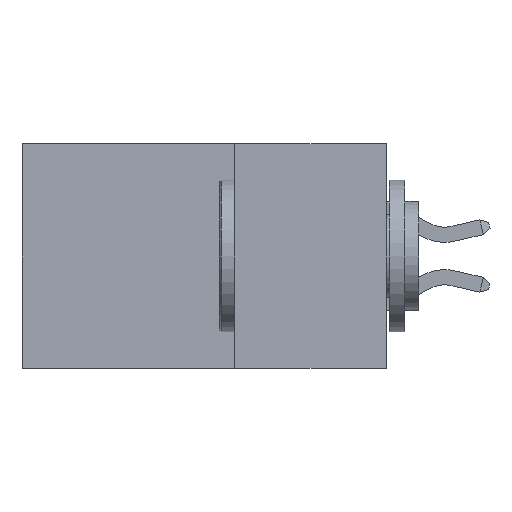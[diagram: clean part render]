
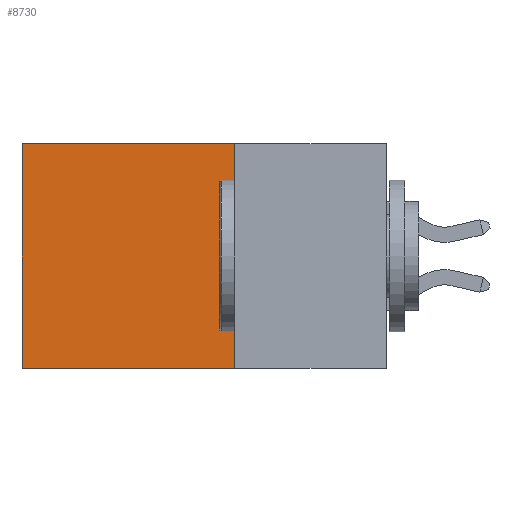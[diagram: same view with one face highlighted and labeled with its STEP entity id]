
A CAD part, left-side view. The second image highlights one B-rep face of the part: STEP entity #8730.
In plain terms, the highlighted planar face has unit normal (-1, 0, 0).
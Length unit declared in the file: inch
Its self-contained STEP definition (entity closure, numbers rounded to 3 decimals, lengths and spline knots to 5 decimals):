
#322 = DIRECTION ( 'NONE',  ( 0., 1., 0. ) ) ;
#375 = VERTEX_POINT ( 'NONE', #1977 ) ;
#406 = CARTESIAN_POINT ( 'NONE',  ( 0.2615, 0.6, -0.37 ) ) ;
#632 = CARTESIAN_POINT ( 'NONE',  ( 0.2615, 0.25, -0.37 ) ) ;
#802 = EDGE_CURVE ( 'NONE', #375, #5498, #2279, .T. ) ;
#880 = LINE ( 'NONE', #4490, #8145 ) ;
#1272 = VECTOR ( 'NONE', #6668, 39.37008 ) ;
#1977 = CARTESIAN_POINT ( 'NONE',  ( 0.2615, 0.25, 0. ) ) ;
#2279 = LINE ( 'NONE', #7722, #9411 ) ;
#2339 = EDGE_LOOP ( 'NONE', ( #3555, #2948, #3907, #2997 ) ) ;
#2371 = DIRECTION ( 'NONE',  ( 1., 0., 0. ) ) ;
#2948 = ORIENTED_EDGE ( 'NONE', *, *, #8869, .F. ) ;
#2973 = CARTESIAN_POINT ( 'NONE',  ( 0.2615, 0.25, -0.37 ) ) ;
#2997 = ORIENTED_EDGE ( 'NONE', *, *, #4298, .T. ) ;
#3555 = ORIENTED_EDGE ( 'NONE', *, *, #7502, .T. ) ;
#3589 = CARTESIAN_POINT ( 'NONE',  ( 0.2615, 0.25, 0. ) ) ;
#3907 = ORIENTED_EDGE ( 'NONE', *, *, #802, .F. ) ;
#4298 = EDGE_CURVE ( 'NONE', #375, #4330, #7429, .T. ) ;
#4330 = VERTEX_POINT ( 'NONE', #9043 ) ;
#4490 = CARTESIAN_POINT ( 'NONE',  ( 0.2615, 0.6, -0.37 ) ) ;
#5498 = VERTEX_POINT ( 'NONE', #2973 ) ;
#5640 = VECTOR ( 'NONE', #322, 39.37008 ) ;
#5743 = AXIS2_PLACEMENT_3D ( 'NONE', #632, #2371, #7263 ) ;
#5896 = PLANE ( 'NONE',  #5743 ) ;
#6194 = DIRECTION ( 'NONE',  ( 0., 0., -1. ) ) ;
#6668 = DIRECTION ( 'NONE',  ( 0., 1., 0. ) ) ;
#7087 = LINE ( 'NONE', #7967, #1272 ) ;
#7198 = DIRECTION ( 'NONE',  ( 0., 0., -1. ) ) ;
#7263 = DIRECTION ( 'NONE',  ( 0., 0., -1. ) ) ;
#7429 = LINE ( 'NONE', #3589, #5640 ) ;
#7502 = EDGE_CURVE ( 'NONE', #4330, #8454, #880, .T. ) ;
#7722 = CARTESIAN_POINT ( 'NONE',  ( 0.2615, 0.25, -0.37 ) ) ;
#7967 = CARTESIAN_POINT ( 'NONE',  ( 0.2615, 0.25, -0.37 ) ) ;
#8145 = VECTOR ( 'NONE', #7198, 39.37008 ) ;
#8454 = VERTEX_POINT ( 'NONE', #406 ) ;
#8730 = ADVANCED_FACE ( 'NONE', ( #9288 ), #5896, .F. ) ;
#8869 = EDGE_CURVE ( 'NONE', #5498, #8454, #7087, .T. ) ;
#9043 = CARTESIAN_POINT ( 'NONE',  ( 0.2615, 0.6, 0. ) ) ;
#9288 = FACE_OUTER_BOUND ( 'NONE', #2339, .T. ) ;
#9411 = VECTOR ( 'NONE', #6194, 39.37008 ) ;
